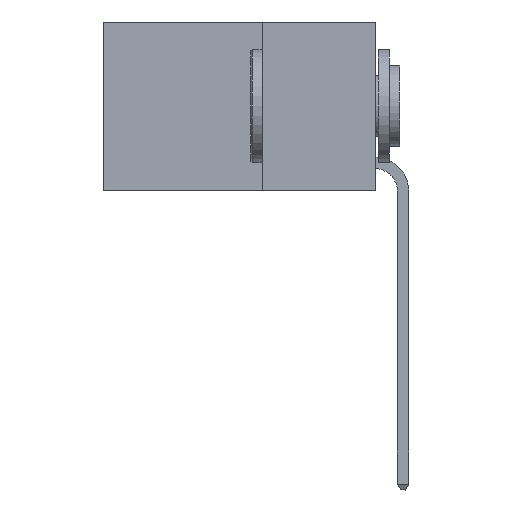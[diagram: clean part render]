
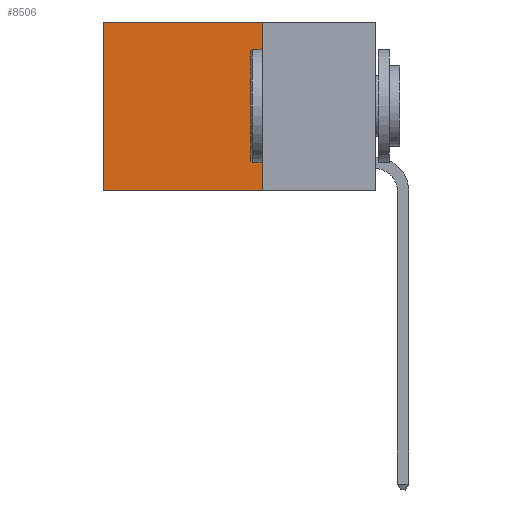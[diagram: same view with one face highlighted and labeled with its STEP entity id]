
A CAD part, left-side view. The second image highlights one B-rep face of the part: STEP entity #8506.
In plain terms, the highlighted planar face has unit normal (-1, 0, 0).
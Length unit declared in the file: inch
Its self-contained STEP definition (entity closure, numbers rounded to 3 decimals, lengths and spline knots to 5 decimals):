
#136 = CARTESIAN_POINT ( 'NONE',  ( 0.2625, 0.6, 0. ) ) ;
#719 = DIRECTION ( 'NONE',  ( 0., 0., -1. ) ) ;
#988 = AXIS2_PLACEMENT_3D ( 'NONE', #6136, #14419, #7417 ) ;
#1566 = LINE ( 'NONE', #15219, #8206 ) ;
#2033 = VECTOR ( 'NONE', #14392, 39.37008 ) ;
#2628 = CARTESIAN_POINT ( 'NONE',  ( 0.2625, 0.25, -0.37 ) ) ;
#3246 = VECTOR ( 'NONE', #14761, 39.37008 ) ;
#3369 = ORIENTED_EDGE ( 'NONE', *, *, #9419, .T. ) ;
#4881 = EDGE_CURVE ( 'NONE', #11164, #13938, #11123, .T. ) ;
#4973 = ORIENTED_EDGE ( 'NONE', *, *, #4881, .F. ) ;
#5352 = CARTESIAN_POINT ( 'NONE',  ( 0.2625, 0.6, -0.37 ) ) ;
#6136 = CARTESIAN_POINT ( 'NONE',  ( 0.2625, 0.25, 0. ) ) ;
#6159 = CARTESIAN_POINT ( 'NONE',  ( 0.2625, 0.25, 0. ) ) ;
#6197 = PLANE ( 'NONE',  #988 ) ;
#6620 = CARTESIAN_POINT ( 'NONE',  ( 0.2625, 0.25, 0. ) ) ;
#6666 = EDGE_CURVE ( 'NONE', #12492, #11164, #9753, .T. ) ;
#7053 = DIRECTION ( 'NONE',  ( 0., 1., 0. ) ) ;
#7228 = VERTEX_POINT ( 'NONE', #136 ) ;
#7232 = CARTESIAN_POINT ( 'NONE',  ( 0.2625, 0.25, -0.37 ) ) ;
#7417 = DIRECTION ( 'NONE',  ( 0., 0., -1. ) ) ;
#7480 = FACE_OUTER_BOUND ( 'NONE', #11129, .T. ) ;
#7889 = CARTESIAN_POINT ( 'NONE',  ( 0.2625, 0.25, 0. ) ) ;
#8206 = VECTOR ( 'NONE', #719, 39.37008 ) ;
#8506 = ADVANCED_FACE ( 'NONE', ( #7480 ), #6197, .F. ) ;
#8635 = LINE ( 'NONE', #6159, #2033 ) ;
#8938 = ORIENTED_EDGE ( 'NONE', *, *, #6666, .F. ) ;
#9419 = EDGE_CURVE ( 'NONE', #7228, #13938, #1566, .T. ) ;
#9753 = LINE ( 'NONE', #6620, #3246 ) ;
#10360 = EDGE_CURVE ( 'NONE', #12492, #7228, #8635, .T. ) ;
#11123 = LINE ( 'NONE', #7232, #11485 ) ;
#11129 = EDGE_LOOP ( 'NONE', ( #3369, #4973, #8938, #13485 ) ) ;
#11164 = VERTEX_POINT ( 'NONE', #2628 ) ;
#11485 = VECTOR ( 'NONE', #7053, 39.37008 ) ;
#12492 = VERTEX_POINT ( 'NONE', #7889 ) ;
#13485 = ORIENTED_EDGE ( 'NONE', *, *, #10360, .T. ) ;
#13938 = VERTEX_POINT ( 'NONE', #5352 ) ;
#14392 = DIRECTION ( 'NONE',  ( 0., 1., 0. ) ) ;
#14419 = DIRECTION ( 'NONE',  ( 1., 0., 0. ) ) ;
#14761 = DIRECTION ( 'NONE',  ( 0., 0., -1. ) ) ;
#15219 = CARTESIAN_POINT ( 'NONE',  ( 0.2625, 0.6, 0. ) ) ;
